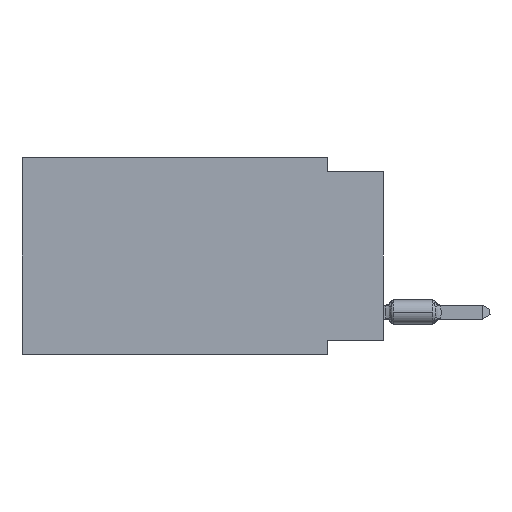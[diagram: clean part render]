
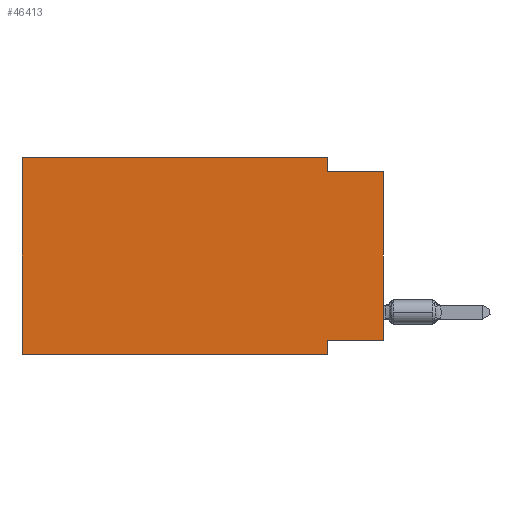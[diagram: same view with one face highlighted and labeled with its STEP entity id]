
A CAD part, left-side view. The second image highlights one B-rep face of the part: STEP entity #46413.
In plain terms, the highlighted planar face has unit normal (-1, 0, 0).
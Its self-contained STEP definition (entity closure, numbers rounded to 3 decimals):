
#2873 = VECTOR ( 'NONE', #36291, 1000. ) ;
#2938 = DIRECTION ( 'NONE',  ( 0., 1., 0. ) ) ;
#3889 = VECTOR ( 'NONE', #53775, 1000. ) ;
#5707 = ORIENTED_EDGE ( 'NONE', *, *, #32751, .T. ) ;
#9447 = LINE ( 'NONE', #59437, #23002 ) ;
#10272 = VERTEX_POINT ( 'NONE', #42590 ) ;
#10683 = EDGE_CURVE ( 'NONE', #32570, #64878, #22322, .T. ) ;
#12266 = CARTESIAN_POINT ( 'NONE',  ( 0., 16.383, 0. ) ) ;
#12607 = DIRECTION ( 'NONE',  ( 0., 0., -1. ) ) ;
#14477 = DIRECTION ( 'NONE',  ( 0., 0., 1. ) ) ;
#15493 = LINE ( 'NONE', #42294, #2873 ) ;
#17900 = CARTESIAN_POINT ( 'NONE',  ( 0., 2.54, -8.89 ) ) ;
#18790 = EDGE_CURVE ( 'NONE', #35295, #51890, #32500, .T. ) ;
#21320 = CARTESIAN_POINT ( 'NONE',  ( 0., 2.54, -8.89 ) ) ;
#21364 = DIRECTION ( 'NONE',  ( 0., -1., 0. ) ) ;
#22322 = LINE ( 'NONE', #53819, #49028 ) ;
#22676 = DIRECTION ( 'NONE',  ( 1., 0., 0. ) ) ;
#23002 = VECTOR ( 'NONE', #14477, 1000. ) ;
#23577 = VERTEX_POINT ( 'NONE', #21320 ) ;
#24782 = CARTESIAN_POINT ( 'NONE',  ( 0., 0., -0.635 ) ) ;
#25413 = LINE ( 'NONE', #45856, #55388 ) ;
#25950 = VERTEX_POINT ( 'NONE', #28644 ) ;
#27714 = FACE_OUTER_BOUND ( 'NONE', #54996, .T. ) ;
#28026 = PLANE ( 'NONE',  #38458 ) ;
#28644 = CARTESIAN_POINT ( 'NONE',  ( 0., 2.54, 0. ) ) ;
#31184 = ORIENTED_EDGE ( 'NONE', *, *, #36879, .F. ) ;
#31346 = LINE ( 'NONE', #17900, #3889 ) ;
#32082 = CARTESIAN_POINT ( 'NONE',  ( 0., 16.383, -8.89 ) ) ;
#32292 = EDGE_CURVE ( 'NONE', #35295, #64878, #38599, .T. ) ;
#32500 = LINE ( 'NONE', #64001, #62661 ) ;
#32570 = VERTEX_POINT ( 'NONE', #64334 ) ;
#32751 = EDGE_CURVE ( 'NONE', #53242, #23577, #15493, .T. ) ;
#34727 = EDGE_CURVE ( 'NONE', #25950, #32570, #59115, .T. ) ;
#35239 = CARTESIAN_POINT ( 'NONE',  ( 0., 0., 0. ) ) ;
#35295 = VERTEX_POINT ( 'NONE', #49478 ) ;
#35531 = ORIENTED_EDGE ( 'NONE', *, *, #10683, .F. ) ;
#36291 = DIRECTION ( 'NONE',  ( 0., -1., 0. ) ) ;
#36879 = EDGE_CURVE ( 'NONE', #51890, #23577, #31346, .T. ) ;
#38458 = AXIS2_PLACEMENT_3D ( 'NONE', #12266, #22676, #12607 ) ;
#38599 = LINE ( 'NONE', #35239, #40324 ) ;
#39264 = ORIENTED_EDGE ( 'NONE', *, *, #32292, .T. ) ;
#39975 = ORIENTED_EDGE ( 'NONE', *, *, #34727, .F. ) ;
#40324 = VECTOR ( 'NONE', #50641, 1000. ) ;
#42294 = CARTESIAN_POINT ( 'NONE',  ( 0., 16.383, -8.89 ) ) ;
#42590 = CARTESIAN_POINT ( 'NONE',  ( 0., 16.383, 0. ) ) ;
#45014 = CARTESIAN_POINT ( 'NONE',  ( 0., 2.54, 0. ) ) ;
#45856 = CARTESIAN_POINT ( 'NONE',  ( 0., 16.383, 0. ) ) ;
#46413 = ADVANCED_FACE ( 'NONE', ( #27714 ), #28026, .F. ) ;
#47551 = ORIENTED_EDGE ( 'NONE', *, *, #53869, .F. ) ;
#48448 = DIRECTION ( 'NONE',  ( 0., -1., 0. ) ) ;
#48454 = ORIENTED_EDGE ( 'NONE', *, *, #51946, .F. ) ;
#49028 = VECTOR ( 'NONE', #48448, 1000. ) ;
#49478 = CARTESIAN_POINT ( 'NONE',  ( 0., 0., -8.255 ) ) ;
#50641 = DIRECTION ( 'NONE',  ( 0., 0., 1. ) ) ;
#51890 = VERTEX_POINT ( 'NONE', #57219 ) ;
#51946 = EDGE_CURVE ( 'NONE', #10272, #25950, #25413, .T. ) ;
#53242 = VERTEX_POINT ( 'NONE', #32082 ) ;
#53775 = DIRECTION ( 'NONE',  ( 0., 0., -1. ) ) ;
#53819 = CARTESIAN_POINT ( 'NONE',  ( 0., 0., -0.635 ) ) ;
#53869 = EDGE_CURVE ( 'NONE', #53242, #10272, #9447, .T. ) ;
#54996 = EDGE_LOOP ( 'NONE', ( #39264, #35531, #39975, #48454, #47551, #5707, #31184, #58448 ) ) ;
#55388 = VECTOR ( 'NONE', #21364, 1000. ) ;
#57219 = CARTESIAN_POINT ( 'NONE',  ( 0., 2.54, -8.255 ) ) ;
#58448 = ORIENTED_EDGE ( 'NONE', *, *, #18790, .F. ) ;
#59115 = LINE ( 'NONE', #45014, #61813 ) ;
#59437 = CARTESIAN_POINT ( 'NONE',  ( 0., 16.383, 0. ) ) ;
#59448 = DIRECTION ( 'NONE',  ( 0., 0., -1. ) ) ;
#61813 = VECTOR ( 'NONE', #59448, 1000. ) ;
#62661 = VECTOR ( 'NONE', #2938, 1000. ) ;
#64001 = CARTESIAN_POINT ( 'NONE',  ( 0., 0., -8.255 ) ) ;
#64334 = CARTESIAN_POINT ( 'NONE',  ( 0., 2.54, -0.635 ) ) ;
#64878 = VERTEX_POINT ( 'NONE', #24782 ) ;
